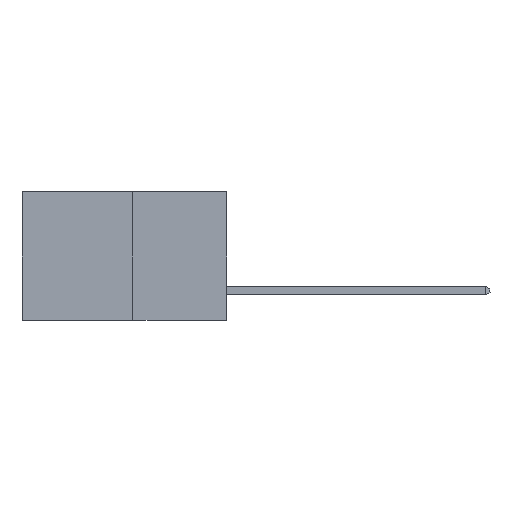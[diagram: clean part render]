
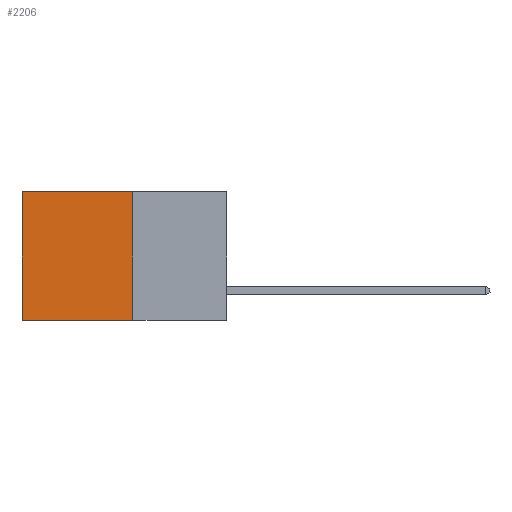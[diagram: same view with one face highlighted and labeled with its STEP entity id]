
A CAD part, left-side view. The second image highlights one B-rep face of the part: STEP entity #2206.
In plain terms, the highlighted planar face has unit normal (-1, 0, 0).
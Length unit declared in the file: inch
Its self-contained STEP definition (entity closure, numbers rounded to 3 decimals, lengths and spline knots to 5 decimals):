
#129 = CARTESIAN_POINT ( 'NONE',  ( 0.277, 0.27, -0.37 ) ) ;
#250 = DIRECTION ( 'NONE',  ( 0., 0., -1. ) ) ;
#460 = ORIENTED_EDGE ( 'NONE', *, *, #6092, .T. ) ;
#602 = CARTESIAN_POINT ( 'NONE',  ( 0.277, 0.59, -0.37 ) ) ;
#837 = AXIS2_PLACEMENT_3D ( 'NONE', #9532, #9350, #1777 ) ;
#1287 = CARTESIAN_POINT ( 'NONE',  ( 0.277, 0.59, 0. ) ) ;
#1457 = CARTESIAN_POINT ( 'NONE',  ( 0.277, 0.59, -0.37 ) ) ;
#1577 = CARTESIAN_POINT ( 'NONE',  ( 0.277, 0.27, -0.37 ) ) ;
#1629 = VERTEX_POINT ( 'NONE', #1287 ) ;
#1777 = DIRECTION ( 'NONE',  ( 0., 0., -1. ) ) ;
#1782 = LINE ( 'NONE', #9910, #4418 ) ;
#2012 = DIRECTION ( 'NONE',  ( 0., 0., -1. ) ) ;
#2206 = ADVANCED_FACE ( 'NONE', ( #4780 ), #9570, .F. ) ;
#2566 = VERTEX_POINT ( 'NONE', #10645 ) ;
#3397 = DIRECTION ( 'NONE',  ( 0., 1., 0. ) ) ;
#3738 = VECTOR ( 'NONE', #10921, 39.37008 ) ;
#4031 = LINE ( 'NONE', #9902, #3738 ) ;
#4418 = VECTOR ( 'NONE', #3397, 39.37008 ) ;
#4780 = FACE_OUTER_BOUND ( 'NONE', #5231, .T. ) ;
#5231 = EDGE_LOOP ( 'NONE', ( #460, #8803, #6602, #6854 ) ) ;
#6092 = EDGE_CURVE ( 'NONE', #1629, #9398, #6528, .T. ) ;
#6528 = LINE ( 'NONE', #602, #10562 ) ;
#6538 = EDGE_CURVE ( 'NONE', #2566, #1629, #4031, .T. ) ;
#6602 = ORIENTED_EDGE ( 'NONE', *, *, #9812, .F. ) ;
#6854 = ORIENTED_EDGE ( 'NONE', *, *, #6538, .T. ) ;
#7934 = VECTOR ( 'NONE', #2012, 39.37008 ) ;
#8382 = VERTEX_POINT ( 'NONE', #1577 ) ;
#8803 = ORIENTED_EDGE ( 'NONE', *, *, #10015, .F. ) ;
#9350 = DIRECTION ( 'NONE',  ( 1., 0., 0. ) ) ;
#9398 = VERTEX_POINT ( 'NONE', #1457 ) ;
#9532 = CARTESIAN_POINT ( 'NONE',  ( 0.277, 0.27, -0.37 ) ) ;
#9570 = PLANE ( 'NONE',  #837 ) ;
#9812 = EDGE_CURVE ( 'NONE', #2566, #8382, #10049, .T. ) ;
#9902 = CARTESIAN_POINT ( 'NONE',  ( 0.277, 0.27, 0. ) ) ;
#9910 = CARTESIAN_POINT ( 'NONE',  ( 0.277, 0.27, -0.37 ) ) ;
#10015 = EDGE_CURVE ( 'NONE', #8382, #9398, #1782, .T. ) ;
#10049 = LINE ( 'NONE', #129, #7934 ) ;
#10562 = VECTOR ( 'NONE', #250, 39.37008 ) ;
#10645 = CARTESIAN_POINT ( 'NONE',  ( 0.277, 0.27, 0. ) ) ;
#10921 = DIRECTION ( 'NONE',  ( 0., 1., 0. ) ) ;
